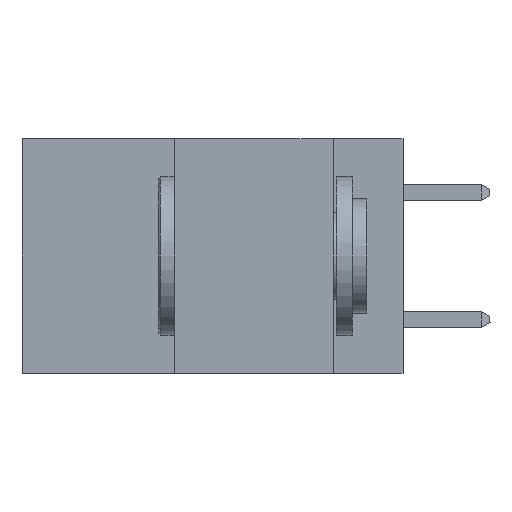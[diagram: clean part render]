
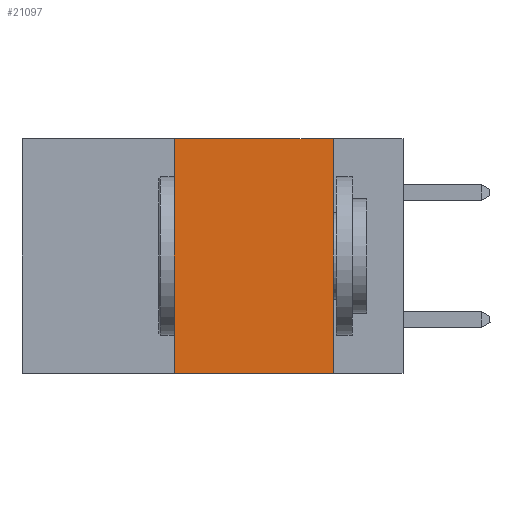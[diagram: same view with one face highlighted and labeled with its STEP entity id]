
A CAD part, left-side view. The second image highlights one B-rep face of the part: STEP entity #21097.
In plain terms, the highlighted planar face has unit normal (-1, 0, 0).
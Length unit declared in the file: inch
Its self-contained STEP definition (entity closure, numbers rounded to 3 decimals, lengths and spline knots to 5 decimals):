
#307 = VERTEX_POINT ( 'NONE', #5992 ) ;
#644 = EDGE_CURVE ( 'NONE', #15244, #307, #3876, .T. ) ;
#659 = EDGE_CURVE ( 'NONE', #1456, #15244, #18075, .T. ) ;
#823 = FACE_OUTER_BOUND ( 'NONE', #18957, .T. ) ;
#1456 = VERTEX_POINT ( 'NONE', #1812 ) ;
#1812 = CARTESIAN_POINT ( 'NONE',  ( 0., 0.36, -0.37 ) ) ;
#3873 = EDGE_CURVE ( 'NONE', #307, #11037, #16703, .T. ) ;
#3876 = LINE ( 'NONE', #21246, #8632 ) ;
#4348 = VECTOR ( 'NONE', #22004, 39.37008 ) ;
#4871 = CARTESIAN_POINT ( 'NONE',  ( 0., 0.36, 0. ) ) ;
#5084 = DIRECTION ( 'NONE',  ( 0., 0., -1. ) ) ;
#5178 = PLANE ( 'NONE',  #14581 ) ;
#5992 = CARTESIAN_POINT ( 'NONE',  ( 0., 0.11, 0. ) ) ;
#6192 = CARTESIAN_POINT ( 'NONE',  ( 0., 0.11, -0.37 ) ) ;
#6795 = ORIENTED_EDGE ( 'NONE', *, *, #659, .F. ) ;
#8471 = EDGE_CURVE ( 'NONE', #1456, #11037, #13537, .T. ) ;
#8632 = VECTOR ( 'NONE', #13696, 39.37008 ) ;
#9352 = CARTESIAN_POINT ( 'NONE',  ( 0., 0.36, 0. ) ) ;
#11037 = VERTEX_POINT ( 'NONE', #6192 ) ;
#12236 = CARTESIAN_POINT ( 'NONE',  ( 0., 0.11, 0. ) ) ;
#12753 = VECTOR ( 'NONE', #13564, 39.37008 ) ;
#13221 = DIRECTION ( 'NONE',  ( 1., 0., 0. ) ) ;
#13537 = LINE ( 'NONE', #21919, #4348 ) ;
#13564 = DIRECTION ( 'NONE',  ( 0., 0., 1. ) ) ;
#13696 = DIRECTION ( 'NONE',  ( 0., -1., 0. ) ) ;
#14396 = ORIENTED_EDGE ( 'NONE', *, *, #3873, .F. ) ;
#14581 = AXIS2_PLACEMENT_3D ( 'NONE', #25301, #13221, #5084 ) ;
#14743 = VECTOR ( 'NONE', #22298, 39.37008 ) ;
#15244 = VERTEX_POINT ( 'NONE', #4871 ) ;
#16703 = LINE ( 'NONE', #12236, #14743 ) ;
#17986 = ORIENTED_EDGE ( 'NONE', *, *, #8471, .T. ) ;
#18075 = LINE ( 'NONE', #9352, #12753 ) ;
#18957 = EDGE_LOOP ( 'NONE', ( #14396, #25677, #6795, #17986 ) ) ;
#21097 = ADVANCED_FACE ( 'NONE', ( #823 ), #5178, .F. ) ;
#21246 = CARTESIAN_POINT ( 'NONE',  ( 0., 0.6, 0. ) ) ;
#21919 = CARTESIAN_POINT ( 'NONE',  ( 0., 0.6, -0.37 ) ) ;
#22004 = DIRECTION ( 'NONE',  ( 0., -1., 0. ) ) ;
#22298 = DIRECTION ( 'NONE',  ( 0., 0., -1. ) ) ;
#25301 = CARTESIAN_POINT ( 'NONE',  ( 0., 0.6, 0. ) ) ;
#25677 = ORIENTED_EDGE ( 'NONE', *, *, #644, .F. ) ;
